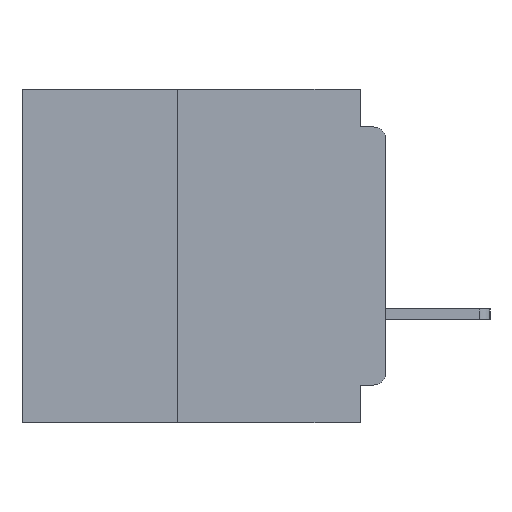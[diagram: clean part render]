
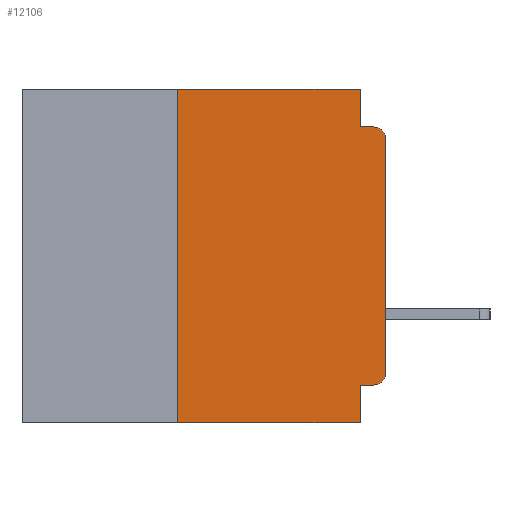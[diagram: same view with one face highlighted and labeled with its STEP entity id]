
A CAD part, left-side view. The second image highlights one B-rep face of the part: STEP entity #12106.
In plain terms, the highlighted planar face has unit normal (-1, 0, 0).
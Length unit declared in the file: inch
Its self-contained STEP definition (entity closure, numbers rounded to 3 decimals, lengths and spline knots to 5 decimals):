
#354 = DIRECTION ( 'NONE',  ( -1., 0., 0. ) ) ;
#369 = CARTESIAN_POINT ( 'NONE',  ( 0., 0.437, 0. ) ) ;
#662 = LINE ( 'NONE', #10363, #21804 ) ;
#3091 = DIRECTION ( 'NONE',  ( 0., 0., -1. ) ) ;
#3353 = EDGE_CURVE ( 'NONE', #8029, #19460, #24308, .T. ) ;
#5208 = CARTESIAN_POINT ( 'NONE',  ( 0., 0.031, 0. ) ) ;
#6059 = VERTEX_POINT ( 'NONE', #48476 ) ;
#6208 = EDGE_CURVE ( 'NONE', #8029, #52416, #13944, .T. ) ;
#6348 = ORIENTED_EDGE ( 'NONE', *, *, #27512, .F. ) ;
#6370 = VERTEX_POINT ( 'NONE', #8808 ) ;
#7148 = AXIS2_PLACEMENT_3D ( 'NONE', #43313, #18432, #47425 ) ;
#8029 = VERTEX_POINT ( 'NONE', #15807 ) ;
#8808 = CARTESIAN_POINT ( 'NONE',  ( 0., 0.015, -0.045 ) ) ;
#9491 = DIRECTION ( 'NONE',  ( 0., 0., -1. ) ) ;
#10363 = CARTESIAN_POINT ( 'NONE',  ( 0., 0., -0.045 ) ) ;
#10936 = VERTEX_POINT ( 'NONE', #52652 ) ;
#11916 = EDGE_CURVE ( 'NONE', #53947, #21961, #20245, .T. ) ;
#12106 = ADVANCED_FACE ( 'NONE', ( #12341 ), #39904, .F. ) ;
#12304 = EDGE_CURVE ( 'NONE', #50513, #28169, #35157, .T. ) ;
#12341 = FACE_OUTER_BOUND ( 'NONE', #25614, .T. ) ;
#12667 = LINE ( 'NONE', #32251, #21197 ) ;
#13635 = CARTESIAN_POINT ( 'NONE',  ( 0., 0.031, -0.045 ) ) ;
#13944 = LINE ( 'NONE', #37128, #26368 ) ;
#14585 = DIRECTION ( 'NONE',  ( 0., -1., 0. ) ) ;
#14987 = DIRECTION ( 'NONE',  ( 1., 0., 0. ) ) ;
#15807 = CARTESIAN_POINT ( 'NONE',  ( 0., 0.25, -0.4 ) ) ;
#16769 = CARTESIAN_POINT ( 'NONE',  ( 0., 0., -0.355 ) ) ;
#18432 = DIRECTION ( 'NONE',  ( -1., 0., 0. ) ) ;
#19401 = CARTESIAN_POINT ( 'NONE',  ( 0., 0., -0.34 ) ) ;
#19460 = VERTEX_POINT ( 'NONE', #42082 ) ;
#19692 = EDGE_CURVE ( 'NONE', #21961, #6370, #662, .T. ) ;
#19752 = LINE ( 'NONE', #40312, #40540 ) ;
#20245 = LINE ( 'NONE', #5208, #51963 ) ;
#20546 = CARTESIAN_POINT ( 'NONE',  ( 0., 0.25, 0. ) ) ;
#21197 = VECTOR ( 'NONE', #3091, 39.37008 ) ;
#21804 = VECTOR ( 'NONE', #14585, 39.37008 ) ;
#21961 = VERTEX_POINT ( 'NONE', #13635 ) ;
#22287 = CARTESIAN_POINT ( 'NONE',  ( 0., 0.437, -0.4 ) ) ;
#22335 = LINE ( 'NONE', #16769, #43105 ) ;
#24308 = LINE ( 'NONE', #22287, #45049 ) ;
#25556 = CARTESIAN_POINT ( 'NONE',  ( 0., 0.015, -0.34 ) ) ;
#25614 = EDGE_LOOP ( 'NONE', ( #28529, #31931, #29991, #49825, #6348, #53709, #46008, #47850, #30583, #51193 ) ) ;
#26368 = VECTOR ( 'NONE', #28784, 39.37008 ) ;
#26481 = DIRECTION ( 'NONE',  ( 0., -1., 0. ) ) ;
#26727 = LINE ( 'NONE', #369, #35168 ) ;
#27512 = EDGE_CURVE ( 'NONE', #52416, #53947, #26727, .T. ) ;
#28169 = VERTEX_POINT ( 'NONE', #19401 ) ;
#28467 = AXIS2_PLACEMENT_3D ( 'NONE', #25556, #354, #29767 ) ;
#28529 = ORIENTED_EDGE ( 'NONE', *, *, #47459, .T. ) ;
#28784 = DIRECTION ( 'NONE',  ( 0., 0., 1. ) ) ;
#29767 = DIRECTION ( 'NONE',  ( 0., 0., -1. ) ) ;
#29991 = ORIENTED_EDGE ( 'NONE', *, *, #19692, .F. ) ;
#30583 = ORIENTED_EDGE ( 'NONE', *, *, #37446, .F. ) ;
#31579 = CARTESIAN_POINT ( 'NONE',  ( 0., 0.437, 0. ) ) ;
#31863 = EDGE_CURVE ( 'NONE', #10936, #6370, #42119, .T. ) ;
#31931 = ORIENTED_EDGE ( 'NONE', *, *, #31863, .T. ) ;
#32251 = CARTESIAN_POINT ( 'NONE',  ( 0., 0.031, -0.4 ) ) ;
#33511 = DIRECTION ( 'NONE',  ( 0., 1., 0. ) ) ;
#33830 = CARTESIAN_POINT ( 'NONE',  ( 0., 0.031, 0. ) ) ;
#33937 = DIRECTION ( 'NONE',  ( 0., -1., 0. ) ) ;
#35157 = CIRCLE ( 'NONE', #28467, 0.015 ) ;
#35168 = VECTOR ( 'NONE', #33937, 39.37008 ) ;
#37128 = CARTESIAN_POINT ( 'NONE',  ( 0., 0.25, -0.4 ) ) ;
#37446 = EDGE_CURVE ( 'NONE', #50513, #6059, #22335, .T. ) ;
#39904 = PLANE ( 'NONE',  #43378 ) ;
#40312 = CARTESIAN_POINT ( 'NONE',  ( 0., 0., 0. ) ) ;
#40540 = VECTOR ( 'NONE', #44476, 39.37008 ) ;
#42082 = CARTESIAN_POINT ( 'NONE',  ( 0., 0.031, -0.4 ) ) ;
#42119 = CIRCLE ( 'NONE', #7148, 0.015 ) ;
#43105 = VECTOR ( 'NONE', #33511, 39.37008 ) ;
#43313 = CARTESIAN_POINT ( 'NONE',  ( 0., 0.015, -0.06 ) ) ;
#43378 = AXIS2_PLACEMENT_3D ( 'NONE', #31579, #14987, #44068 ) ;
#43623 = EDGE_CURVE ( 'NONE', #6059, #19460, #12667, .T. ) ;
#44068 = DIRECTION ( 'NONE',  ( 0., 0., -1. ) ) ;
#44476 = DIRECTION ( 'NONE',  ( 0., 0., 1. ) ) ;
#45049 = VECTOR ( 'NONE', #26481, 39.37008 ) ;
#46008 = ORIENTED_EDGE ( 'NONE', *, *, #3353, .T. ) ;
#47425 = DIRECTION ( 'NONE',  ( 0., 0., -1. ) ) ;
#47459 = EDGE_CURVE ( 'NONE', #28169, #10936, #19752, .T. ) ;
#47850 = ORIENTED_EDGE ( 'NONE', *, *, #43623, .F. ) ;
#48476 = CARTESIAN_POINT ( 'NONE',  ( 0., 0.031, -0.355 ) ) ;
#49825 = ORIENTED_EDGE ( 'NONE', *, *, #11916, .F. ) ;
#50513 = VERTEX_POINT ( 'NONE', #52763 ) ;
#51193 = ORIENTED_EDGE ( 'NONE', *, *, #12304, .T. ) ;
#51963 = VECTOR ( 'NONE', #9491, 39.37008 ) ;
#52416 = VERTEX_POINT ( 'NONE', #20546 ) ;
#52652 = CARTESIAN_POINT ( 'NONE',  ( 0., 0., -0.06 ) ) ;
#52763 = CARTESIAN_POINT ( 'NONE',  ( 0., 0.015, -0.355 ) ) ;
#53709 = ORIENTED_EDGE ( 'NONE', *, *, #6208, .F. ) ;
#53947 = VERTEX_POINT ( 'NONE', #33830 ) ;
